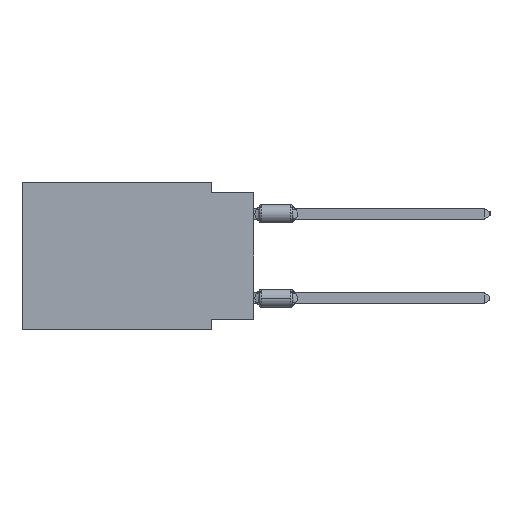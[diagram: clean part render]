
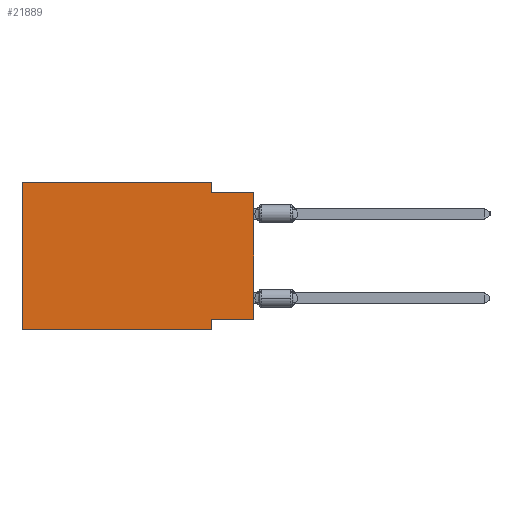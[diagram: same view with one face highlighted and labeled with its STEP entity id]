
A CAD part, left-side view. The second image highlights one B-rep face of the part: STEP entity #21889.
In plain terms, the highlighted planar face has unit normal (-1, 0, 0).
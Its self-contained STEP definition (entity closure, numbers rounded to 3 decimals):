
#181 = CARTESIAN_POINT ( 'NONE',  ( 0., 2.54, 0. ) ) ;
#985 = LINE ( 'NONE', #1165, #2028 ) ;
#1165 = CARTESIAN_POINT ( 'NONE',  ( 0., 13.97, 0. ) ) ;
#1863 = ORIENTED_EDGE ( 'NONE', *, *, #12702, .F. ) ;
#2028 = VECTOR ( 'NONE', #12201, 1000. ) ;
#2107 = DIRECTION ( 'NONE',  ( 0., -1., 0. ) ) ;
#2757 = CARTESIAN_POINT ( 'NONE',  ( 0., 2.54, 0. ) ) ;
#2765 = VECTOR ( 'NONE', #8359, 1000. ) ;
#3130 = VECTOR ( 'NONE', #12346, 1000. ) ;
#3450 = EDGE_CURVE ( 'NONE', #8773, #6691, #8403, .T. ) ;
#3492 = CARTESIAN_POINT ( 'NONE',  ( 0., 2.54, -8.89 ) ) ;
#3767 = CARTESIAN_POINT ( 'NONE',  ( 0., 13.97, 0. ) ) ;
#4751 = VECTOR ( 'NONE', #2107, 1000. ) ;
#5760 = EDGE_CURVE ( 'NONE', #8773, #21145, #18173, .T. ) ;
#6691 = VERTEX_POINT ( 'NONE', #6893 ) ;
#6893 = CARTESIAN_POINT ( 'NONE',  ( 0., 0., -0.635 ) ) ;
#7142 = VERTEX_POINT ( 'NONE', #3767 ) ;
#8359 = DIRECTION ( 'NONE',  ( 0., 1., 0. ) ) ;
#8403 = LINE ( 'NONE', #9119, #30171 ) ;
#8501 = VECTOR ( 'NONE', #35461, 1000. ) ;
#8773 = VERTEX_POINT ( 'NONE', #21404 ) ;
#8830 = CARTESIAN_POINT ( 'NONE',  ( 0., 13.97, 0. ) ) ;
#9119 = CARTESIAN_POINT ( 'NONE',  ( 0., 0., 0. ) ) ;
#9640 = LINE ( 'NONE', #31657, #22833 ) ;
#11358 = FACE_OUTER_BOUND ( 'NONE', #32366, .T. ) ;
#12177 = EDGE_CURVE ( 'NONE', #7142, #14226, #985, .T. ) ;
#12201 = DIRECTION ( 'NONE',  ( 0., -1., 0. ) ) ;
#12346 = DIRECTION ( 'NONE',  ( 0., 0., -1. ) ) ;
#12561 = CARTESIAN_POINT ( 'NONE',  ( 0., 2.54, -8.255 ) ) ;
#12702 = EDGE_CURVE ( 'NONE', #19818, #6691, #9640, .T. ) ;
#13058 = VECTOR ( 'NONE', #13777, 1000. ) ;
#13569 = EDGE_CURVE ( 'NONE', #14092, #21076, #21798, .T. ) ;
#13777 = DIRECTION ( 'NONE',  ( 0., 0., -1. ) ) ;
#13814 = DIRECTION ( 'NONE',  ( 0., 0., 1. ) ) ;
#14092 = VERTEX_POINT ( 'NONE', #33821 ) ;
#14226 = VERTEX_POINT ( 'NONE', #181 ) ;
#15229 = DIRECTION ( 'NONE',  ( 0., -1., 0. ) ) ;
#15691 = ORIENTED_EDGE ( 'NONE', *, *, #12177, .F. ) ;
#17837 = CARTESIAN_POINT ( 'NONE',  ( 0., 13.97, 0. ) ) ;
#18173 = LINE ( 'NONE', #33078, #2765 ) ;
#19456 = EDGE_CURVE ( 'NONE', #14092, #7142, #24444, .T. ) ;
#19596 = CARTESIAN_POINT ( 'NONE',  ( 0., 2.54, -0.635 ) ) ;
#19818 = VERTEX_POINT ( 'NONE', #19596 ) ;
#21076 = VERTEX_POINT ( 'NONE', #32659 ) ;
#21145 = VERTEX_POINT ( 'NONE', #12561 ) ;
#21404 = CARTESIAN_POINT ( 'NONE',  ( 0., 0., -8.255 ) ) ;
#21798 = LINE ( 'NONE', #29551, #4751 ) ;
#21889 = ADVANCED_FACE ( 'NONE', ( #11358 ), #22722, .F. ) ;
#22244 = EDGE_CURVE ( 'NONE', #21145, #21076, #31115, .T. ) ;
#22545 = DIRECTION ( 'NONE',  ( 0., 0., -1. ) ) ;
#22722 = PLANE ( 'NONE',  #31444 ) ;
#22833 = VECTOR ( 'NONE', #15229, 1000. ) ;
#23141 = ORIENTED_EDGE ( 'NONE', *, *, #3450, .T. ) ;
#24444 = LINE ( 'NONE', #17837, #8501 ) ;
#27487 = LINE ( 'NONE', #2757, #13058 ) ;
#28565 = ORIENTED_EDGE ( 'NONE', *, *, #22244, .F. ) ;
#29551 = CARTESIAN_POINT ( 'NONE',  ( 0., 13.97, -8.89 ) ) ;
#30171 = VECTOR ( 'NONE', #13814, 1000. ) ;
#30875 = ORIENTED_EDGE ( 'NONE', *, *, #5760, .F. ) ;
#31026 = DIRECTION ( 'NONE',  ( 1., 0., 0. ) ) ;
#31115 = LINE ( 'NONE', #3492, #3130 ) ;
#31444 = AXIS2_PLACEMENT_3D ( 'NONE', #8830, #31026, #22545 ) ;
#31657 = CARTESIAN_POINT ( 'NONE',  ( 0., 0., -0.635 ) ) ;
#31986 = ORIENTED_EDGE ( 'NONE', *, *, #33130, .F. ) ;
#32366 = EDGE_LOOP ( 'NONE', ( #23141, #1863, #31986, #15691, #34829, #35275, #28565, #30875 ) ) ;
#32659 = CARTESIAN_POINT ( 'NONE',  ( 0., 2.54, -8.89 ) ) ;
#33078 = CARTESIAN_POINT ( 'NONE',  ( 0., 0., -8.255 ) ) ;
#33130 = EDGE_CURVE ( 'NONE', #14226, #19818, #27487, .T. ) ;
#33821 = CARTESIAN_POINT ( 'NONE',  ( 0., 13.97, -8.89 ) ) ;
#34829 = ORIENTED_EDGE ( 'NONE', *, *, #19456, .F. ) ;
#35275 = ORIENTED_EDGE ( 'NONE', *, *, #13569, .T. ) ;
#35461 = DIRECTION ( 'NONE',  ( 0., 0., 1. ) ) ;
